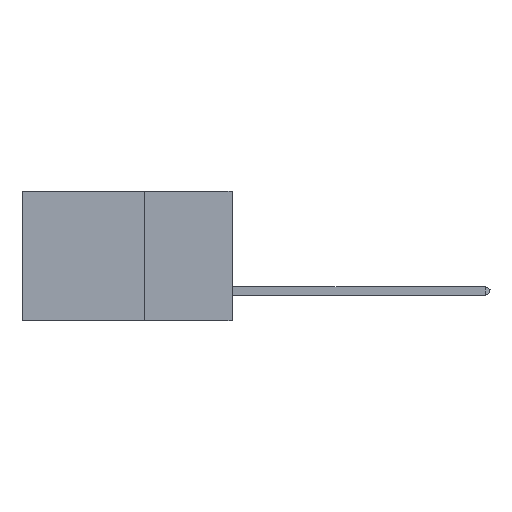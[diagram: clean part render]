
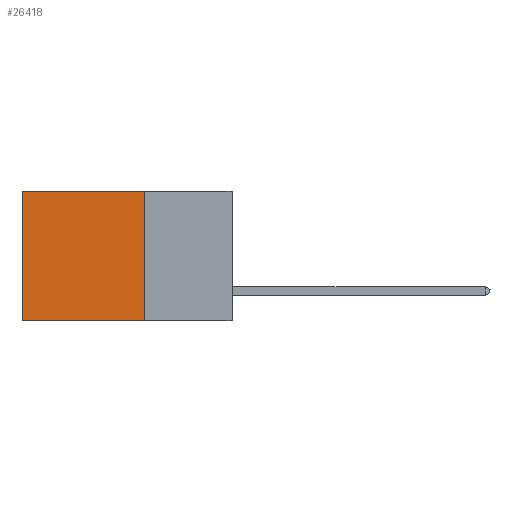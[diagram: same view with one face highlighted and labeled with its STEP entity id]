
A CAD part, left-side view. The second image highlights one B-rep face of the part: STEP entity #26418.
In plain terms, the highlighted planar face has unit normal (-1, 0, 0).
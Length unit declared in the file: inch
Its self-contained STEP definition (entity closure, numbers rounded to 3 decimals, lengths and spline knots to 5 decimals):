
#724 = LINE ( 'NONE', #29975, #19586 ) ;
#1108 = VECTOR ( 'NONE', #33310, 39.37008 ) ;
#1641 = LINE ( 'NONE', #5929, #1108 ) ;
#2680 = DIRECTION ( 'NONE',  ( 0., 0., -1. ) ) ;
#5058 = DIRECTION ( 'NONE',  ( 0., 0., -1. ) ) ;
#5070 = CARTESIAN_POINT ( 'NONE',  ( 0.2875, 0.6, 0. ) ) ;
#5929 = CARTESIAN_POINT ( 'NONE',  ( 0.2875, 0.25, -0.37 ) ) ;
#6649 = VECTOR ( 'NONE', #5058, 39.37008 ) ;
#6729 = DIRECTION ( 'NONE',  ( 1., 0., 0. ) ) ;
#6969 = EDGE_CURVE ( 'NONE', #37508, #7250, #1641, .T. ) ;
#7250 = VERTEX_POINT ( 'NONE', #33981 ) ;
#8613 = FACE_OUTER_BOUND ( 'NONE', #14261, .T. ) ;
#14261 = EDGE_LOOP ( 'NONE', ( #30196, #21789, #32168, #19137 ) ) ;
#19137 = ORIENTED_EDGE ( 'NONE', *, *, #35486, .T. ) ;
#19586 = VECTOR ( 'NONE', #26533, 39.37008 ) ;
#20541 = PLANE ( 'NONE',  #22826 ) ;
#21789 = ORIENTED_EDGE ( 'NONE', *, *, #6969, .F. ) ;
#22195 = CARTESIAN_POINT ( 'NONE',  ( 0.2875, 0.25, 0. ) ) ;
#22826 = AXIS2_PLACEMENT_3D ( 'NONE', #44389, #6729, #2680 ) ;
#26418 = ADVANCED_FACE ( 'NONE', ( #8613 ), #20541, .F. ) ;
#26533 = DIRECTION ( 'NONE',  ( 0., 1., 0. ) ) ;
#28717 = VECTOR ( 'NONE', #30457, 39.37008 ) ;
#29217 = LINE ( 'NONE', #30710, #6649 ) ;
#29975 = CARTESIAN_POINT ( 'NONE',  ( 0.2875, 0.25, 0. ) ) ;
#30196 = ORIENTED_EDGE ( 'NONE', *, *, #31842, .T. ) ;
#30457 = DIRECTION ( 'NONE',  ( 0., 0., -1. ) ) ;
#30535 = CARTESIAN_POINT ( 'NONE',  ( 0.2875, 0.6, 0. ) ) ;
#30710 = CARTESIAN_POINT ( 'NONE',  ( 0.2875, 0.25, 0. ) ) ;
#31842 = EDGE_CURVE ( 'NONE', #33853, #7250, #34637, .T. ) ;
#32168 = ORIENTED_EDGE ( 'NONE', *, *, #35890, .F. ) ;
#33310 = DIRECTION ( 'NONE',  ( 0., 1., 0. ) ) ;
#33853 = VERTEX_POINT ( 'NONE', #30535 ) ;
#33981 = CARTESIAN_POINT ( 'NONE',  ( 0.2875, 0.6, -0.37 ) ) ;
#34637 = LINE ( 'NONE', #5070, #28717 ) ;
#35486 = EDGE_CURVE ( 'NONE', #35938, #33853, #724, .T. ) ;
#35890 = EDGE_CURVE ( 'NONE', #35938, #37508, #29217, .T. ) ;
#35938 = VERTEX_POINT ( 'NONE', #22195 ) ;
#37508 = VERTEX_POINT ( 'NONE', #41739 ) ;
#41739 = CARTESIAN_POINT ( 'NONE',  ( 0.2875, 0.25, -0.37 ) ) ;
#44389 = CARTESIAN_POINT ( 'NONE',  ( 0.2875, 0.25, 0. ) ) ;
